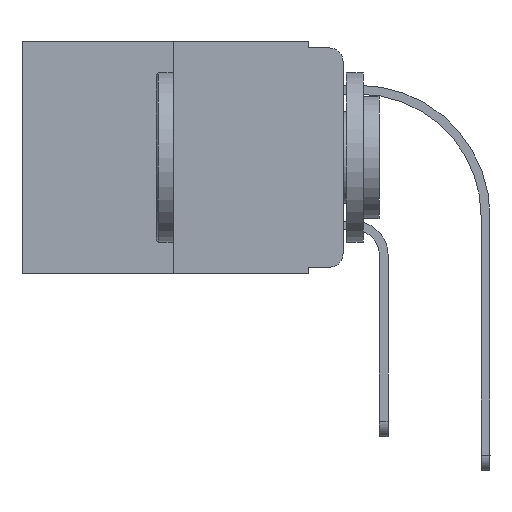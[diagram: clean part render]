
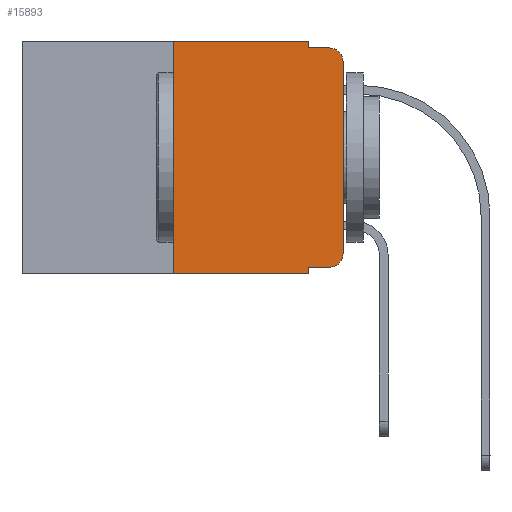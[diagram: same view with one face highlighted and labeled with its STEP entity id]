
A CAD part, left-side view. The second image highlights one B-rep face of the part: STEP entity #15893.
In plain terms, the highlighted planar face has unit normal (-1, 0, 0).
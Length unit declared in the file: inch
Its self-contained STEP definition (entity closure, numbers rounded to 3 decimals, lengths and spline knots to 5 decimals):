
#120 = VERTEX_POINT ( 'NONE', #12441 ) ;
#661 = CARTESIAN_POINT ( 'NONE',  ( 0., 0.051, -0.343 ) ) ;
#901 = CARTESIAN_POINT ( 'NONE',  ( 0., 0., -0.313 ) ) ;
#1138 = CARTESIAN_POINT ( 'NONE',  ( 0., 0.25, 0. ) ) ;
#1393 = CARTESIAN_POINT ( 'NONE',  ( 0., 0.051, 0. ) ) ;
#1683 = VERTEX_POINT ( 'NONE', #1393 ) ;
#1794 = EDGE_CURVE ( 'NONE', #15150, #10758, #3673, .T. ) ;
#1927 = CARTESIAN_POINT ( 'NONE',  ( 0., 0.051, 0. ) ) ;
#2130 = EDGE_CURVE ( 'NONE', #12686, #1683, #10163, .T. ) ;
#2476 = AXIS2_PLACEMENT_3D ( 'NONE', #17712, #2801, #15765 ) ;
#2488 = PLANE ( 'NONE',  #2476 ) ;
#2784 = VERTEX_POINT ( 'NONE', #15903 ) ;
#2801 = DIRECTION ( 'NONE',  ( 1., 0., 0. ) ) ;
#3523 = ORIENTED_EDGE ( 'NONE', *, *, #16138, .T. ) ;
#3578 = DIRECTION ( 'NONE',  ( 0., 0., -1. ) ) ;
#3673 = LINE ( 'NONE', #8555, #7367 ) ;
#3773 = ORIENTED_EDGE ( 'NONE', *, *, #13573, .T. ) ;
#4023 = VERTEX_POINT ( 'NONE', #901 ) ;
#4241 = DIRECTION ( 'NONE',  ( 0., -1., 0. ) ) ;
#4281 = CARTESIAN_POINT ( 'NONE',  ( 0., 0.02, -0.313 ) ) ;
#4630 = CIRCLE ( 'NONE', #19572, 0.02 ) ;
#4819 = CARTESIAN_POINT ( 'NONE',  ( 0., 0., -0.03 ) ) ;
#5081 = DIRECTION ( 'NONE',  ( 0., 0., 1. ) ) ;
#6636 = EDGE_CURVE ( 'NONE', #15150, #12686, #10922, .T. ) ;
#6979 = VECTOR ( 'NONE', #19789, 39.37008 ) ;
#6999 = CARTESIAN_POINT ( 'NONE',  ( 0., 0.473, 0. ) ) ;
#7017 = DIRECTION ( 'NONE',  ( 0., 0., -1. ) ) ;
#7367 = VECTOR ( 'NONE', #15421, 39.37008 ) ;
#7431 = ORIENTED_EDGE ( 'NONE', *, *, #1794, .T. ) ;
#7559 = ORIENTED_EDGE ( 'NONE', *, *, #14834, .F. ) ;
#7628 = VECTOR ( 'NONE', #7017, 39.37008 ) ;
#8332 = ORIENTED_EDGE ( 'NONE', *, *, #17702, .F. ) ;
#8555 = CARTESIAN_POINT ( 'NONE',  ( 0., 0.473, -0.343 ) ) ;
#8677 = DIRECTION ( 'NONE',  ( -1., 0., 0. ) ) ;
#9519 = LINE ( 'NONE', #17796, #12260 ) ;
#10016 = CARTESIAN_POINT ( 'NONE',  ( 0., 0.25, -0.343 ) ) ;
#10163 = LINE ( 'NONE', #6999, #11209 ) ;
#10183 = VERTEX_POINT ( 'NONE', #13626 ) ;
#10758 = VERTEX_POINT ( 'NONE', #661 ) ;
#10916 = DIRECTION ( 'NONE',  ( -1., 0., 0. ) ) ;
#10922 = LINE ( 'NONE', #1138, #15386 ) ;
#11071 = FACE_OUTER_BOUND ( 'NONE', #20945, .T. ) ;
#11209 = VECTOR ( 'NONE', #16819, 39.37008 ) ;
#11270 = DIRECTION ( 'NONE',  ( 0., 0., -1. ) ) ;
#11357 = VERTEX_POINT ( 'NONE', #4819 ) ;
#12260 = VECTOR ( 'NONE', #11270, 39.37008 ) ;
#12441 = CARTESIAN_POINT ( 'NONE',  ( 0., 0.051, -0.333 ) ) ;
#12686 = VERTEX_POINT ( 'NONE', #14643 ) ;
#12840 = AXIS2_PLACEMENT_3D ( 'NONE', #18281, #8677, #3578 ) ;
#13246 = CIRCLE ( 'NONE', #12840, 0.02 ) ;
#13559 = LINE ( 'NONE', #20207, #14624 ) ;
#13573 = EDGE_CURVE ( 'NONE', #120, #10183, #17947, .T. ) ;
#13626 = CARTESIAN_POINT ( 'NONE',  ( 0., 0.02, -0.333 ) ) ;
#13845 = ORIENTED_EDGE ( 'NONE', *, *, #14330, .T. ) ;
#14330 = EDGE_CURVE ( 'NONE', #11357, #2784, #13246, .T. ) ;
#14454 = CARTESIAN_POINT ( 'NONE',  ( 0., 0.051, -0.333 ) ) ;
#14624 = VECTOR ( 'NONE', #5081, 39.37008 ) ;
#14643 = CARTESIAN_POINT ( 'NONE',  ( 0., 0.25, 0. ) ) ;
#14834 = EDGE_CURVE ( 'NONE', #120, #10758, #16948, .T. ) ;
#15019 = ORIENTED_EDGE ( 'NONE', *, *, #19993, .F. ) ;
#15150 = VERTEX_POINT ( 'NONE', #10016 ) ;
#15386 = VECTOR ( 'NONE', #17465, 39.37008 ) ;
#15421 = DIRECTION ( 'NONE',  ( 0., -1., 0. ) ) ;
#15765 = DIRECTION ( 'NONE',  ( 0., 0., -1. ) ) ;
#15878 = ORIENTED_EDGE ( 'NONE', *, *, #2130, .F. ) ;
#15893 = ADVANCED_FACE ( 'NONE', ( #11071 ), #2488, .F. ) ;
#15903 = CARTESIAN_POINT ( 'NONE',  ( 0., 0.02, -0.01 ) ) ;
#16138 = EDGE_CURVE ( 'NONE', #4023, #11357, #13559, .T. ) ;
#16819 = DIRECTION ( 'NONE',  ( 0., -1., 0. ) ) ;
#16948 = LINE ( 'NONE', #1927, #7628 ) ;
#17269 = VERTEX_POINT ( 'NONE', #19672 ) ;
#17465 = DIRECTION ( 'NONE',  ( 0., 0., 1. ) ) ;
#17702 = EDGE_CURVE ( 'NONE', #1683, #17269, #9519, .T. ) ;
#17712 = CARTESIAN_POINT ( 'NONE',  ( 0., 0.473, 0. ) ) ;
#17796 = CARTESIAN_POINT ( 'NONE',  ( 0., 0.051, 0. ) ) ;
#17947 = LINE ( 'NONE', #14454, #6979 ) ;
#18107 = EDGE_CURVE ( 'NONE', #10183, #4023, #4630, .T. ) ;
#18281 = CARTESIAN_POINT ( 'NONE',  ( 0., 0.02, -0.03 ) ) ;
#18874 = DIRECTION ( 'NONE',  ( 0., 0., -1. ) ) ;
#19358 = CARTESIAN_POINT ( 'NONE',  ( 0., 0.051, -0.01 ) ) ;
#19428 = ORIENTED_EDGE ( 'NONE', *, *, #6636, .F. ) ;
#19572 = AXIS2_PLACEMENT_3D ( 'NONE', #4281, #10916, #18874 ) ;
#19672 = CARTESIAN_POINT ( 'NONE',  ( 0., 0.051, -0.01 ) ) ;
#19789 = DIRECTION ( 'NONE',  ( 0., -1., 0. ) ) ;
#19866 = ORIENTED_EDGE ( 'NONE', *, *, #18107, .T. ) ;
#19993 = EDGE_CURVE ( 'NONE', #17269, #2784, #20799, .T. ) ;
#20207 = CARTESIAN_POINT ( 'NONE',  ( 0., 0., 0. ) ) ;
#20799 = LINE ( 'NONE', #19358, #20974 ) ;
#20945 = EDGE_LOOP ( 'NONE', ( #3523, #13845, #15019, #8332, #15878, #19428, #7431, #7559, #3773, #19866 ) ) ;
#20974 = VECTOR ( 'NONE', #4241, 39.37008 ) ;
